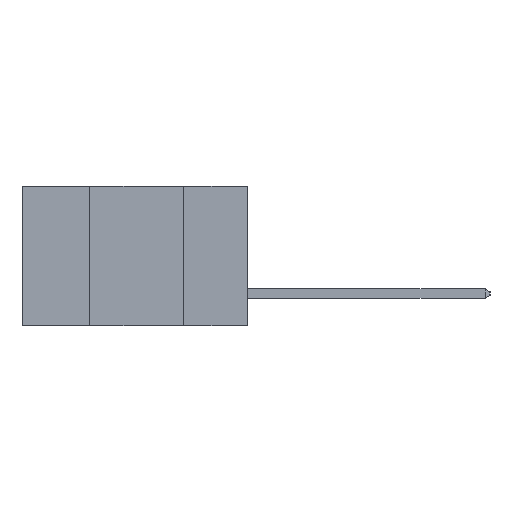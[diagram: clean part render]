
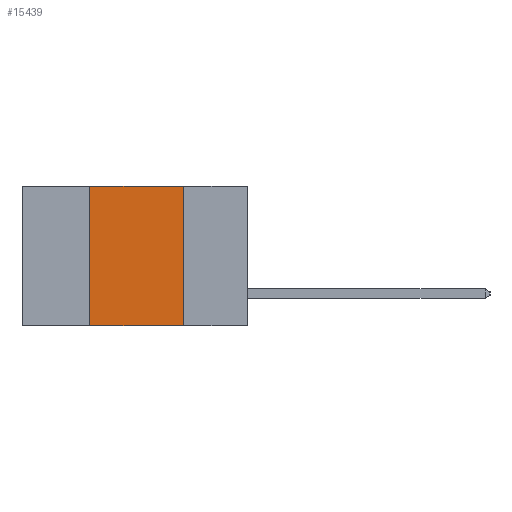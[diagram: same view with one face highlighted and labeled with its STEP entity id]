
A CAD part, left-side view. The second image highlights one B-rep face of the part: STEP entity #15439.
In plain terms, the highlighted planar face has unit normal (-1, 0, 0).
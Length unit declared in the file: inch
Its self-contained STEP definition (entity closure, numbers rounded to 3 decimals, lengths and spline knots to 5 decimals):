
#41 = CARTESIAN_POINT ( 'NONE',  ( 0., 0.42, 0. ) ) ;
#1315 = EDGE_CURVE ( 'NONE', #17129, #6599, #2928, .T. ) ;
#1383 = LINE ( 'NONE', #15039, #16591 ) ;
#1752 = DIRECTION ( 'NONE',  ( 0., 0., -1. ) ) ;
#1994 = DIRECTION ( 'NONE',  ( 0., 0., -1. ) ) ;
#2108 = DIRECTION ( 'NONE',  ( 0., -1., 0. ) ) ;
#2928 = LINE ( 'NONE', #17681, #18129 ) ;
#2995 = LINE ( 'NONE', #9199, #14390 ) ;
#3412 = VECTOR ( 'NONE', #7052, 39.37008 ) ;
#3758 = VERTEX_POINT ( 'NONE', #18417 ) ;
#3863 = CARTESIAN_POINT ( 'NONE',  ( 0., 0.17, 0. ) ) ;
#3966 = EDGE_CURVE ( 'NONE', #10506, #3758, #14777, .T. ) ;
#6599 = VERTEX_POINT ( 'NONE', #3863 ) ;
#7052 = DIRECTION ( 'NONE',  ( 0., -1., 0. ) ) ;
#9024 = EDGE_CURVE ( 'NONE', #10506, #17129, #2995, .T. ) ;
#9199 = CARTESIAN_POINT ( 'NONE',  ( 0., 0.42, 0. ) ) ;
#9254 = PLANE ( 'NONE',  #17706 ) ;
#9717 = ORIENTED_EDGE ( 'NONE', *, *, #1315, .F. ) ;
#10506 = VERTEX_POINT ( 'NONE', #15942 ) ;
#10644 = ORIENTED_EDGE ( 'NONE', *, *, #3966, .T. ) ;
#10674 = CARTESIAN_POINT ( 'NONE',  ( 0., 0.6, 0. ) ) ;
#10740 = DIRECTION ( 'NONE',  ( 1., 0., 0. ) ) ;
#11948 = EDGE_CURVE ( 'NONE', #6599, #3758, #1383, .T. ) ;
#12216 = EDGE_LOOP ( 'NONE', ( #13141, #9717, #17390, #10644 ) ) ;
#13016 = CARTESIAN_POINT ( 'NONE',  ( 0., 0.6, -0.37 ) ) ;
#13141 = ORIENTED_EDGE ( 'NONE', *, *, #11948, .F. ) ;
#13614 = DIRECTION ( 'NONE',  ( 0., 0., 1. ) ) ;
#14390 = VECTOR ( 'NONE', #13614, 39.37008 ) ;
#14777 = LINE ( 'NONE', #13016, #3412 ) ;
#15039 = CARTESIAN_POINT ( 'NONE',  ( 0., 0.17, 0. ) ) ;
#15439 = ADVANCED_FACE ( 'NONE', ( #18741 ), #9254, .F. ) ;
#15942 = CARTESIAN_POINT ( 'NONE',  ( 0., 0.42, -0.37 ) ) ;
#16591 = VECTOR ( 'NONE', #1994, 39.37008 ) ;
#17129 = VERTEX_POINT ( 'NONE', #41 ) ;
#17390 = ORIENTED_EDGE ( 'NONE', *, *, #9024, .F. ) ;
#17681 = CARTESIAN_POINT ( 'NONE',  ( 0., 0.6, 0. ) ) ;
#17706 = AXIS2_PLACEMENT_3D ( 'NONE', #10674, #10740, #1752 ) ;
#18129 = VECTOR ( 'NONE', #2108, 39.37008 ) ;
#18417 = CARTESIAN_POINT ( 'NONE',  ( 0., 0.17, -0.37 ) ) ;
#18741 = FACE_OUTER_BOUND ( 'NONE', #12216, .T. ) ;
